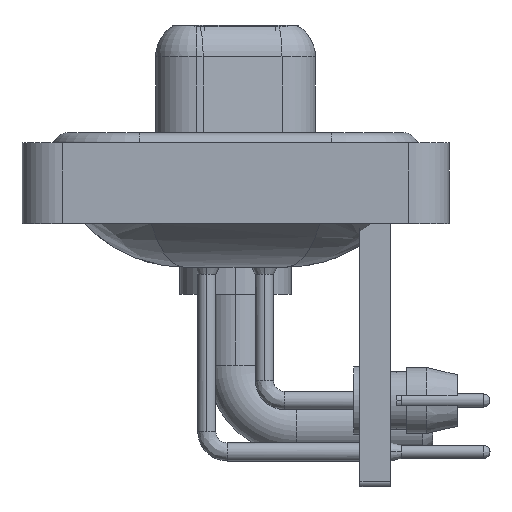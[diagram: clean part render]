
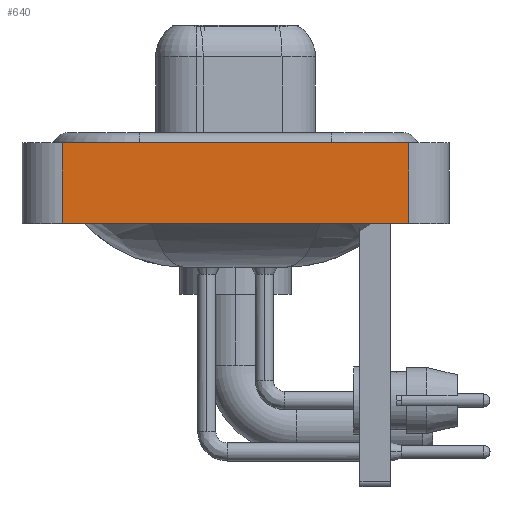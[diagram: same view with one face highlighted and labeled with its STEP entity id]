
A CAD part, left-side view. The second image highlights one B-rep face of the part: STEP entity #640.
In plain terms, the highlighted planar face has unit normal (-1, 0, 0).
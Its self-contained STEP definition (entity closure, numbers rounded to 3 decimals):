
#111 = EDGE_CURVE ( 'NONE', #170, #990, #12064, .T. ) ;
#170 = VERTEX_POINT ( 'NONE', #10015 ) ;
#640 = ADVANCED_FACE ( 'NONE', ( #26534 ), #17726, .T. ) ;
#821 = ORIENTED_EDGE ( 'NONE', *, *, #111, .F. ) ;
#990 = VERTEX_POINT ( 'NONE', #11814 ) ;
#1239 = ORIENTED_EDGE ( 'NONE', *, *, #27075, .T. ) ;
#2678 = VECTOR ( 'NONE', #25420, 1000. ) ;
#3012 = VERTEX_POINT ( 'NONE', #8261 ) ;
#5232 = LINE ( 'NONE', #21174, #9393 ) ;
#5354 = CARTESIAN_POINT ( 'NONE',  ( -7.35, 8.55, -3.6 ) ) ;
#5956 = AXIS2_PLACEMENT_3D ( 'NONE', #17164, #28735, #21721 ) ;
#7904 = VERTEX_POINT ( 'NONE', #26874 ) ;
#8261 = CARTESIAN_POINT ( 'NONE',  ( -7.35, -8.55, -3.6 ) ) ;
#8677 = LINE ( 'NONE', #17750, #10166 ) ;
#8840 = DIRECTION ( 'NONE',  ( 0., -1., 0. ) ) ;
#9393 = VECTOR ( 'NONE', #13995, 1000. ) ;
#10015 = CARTESIAN_POINT ( 'NONE',  ( -7.35, 8.55, -3.6 ) ) ;
#10166 = VECTOR ( 'NONE', #26558, 1000. ) ;
#11035 = LINE ( 'NONE', #19962, #24167 ) ;
#11756 = ORIENTED_EDGE ( 'NONE', *, *, #22994, .F. ) ;
#11814 = CARTESIAN_POINT ( 'NONE',  ( -7.35, 8.55, 0.4 ) ) ;
#12064 = LINE ( 'NONE', #5354, #2678 ) ;
#13995 = DIRECTION ( 'NONE',  ( 0., 0., 1. ) ) ;
#15610 = EDGE_CURVE ( 'NONE', #3012, #7904, #5232, .T. ) ;
#17164 = CARTESIAN_POINT ( 'NONE',  ( -7.35, -8.55, -3.6 ) ) ;
#17726 = PLANE ( 'NONE',  #5956 ) ;
#17750 = CARTESIAN_POINT ( 'NONE',  ( -7.35, -8.55, -3.6 ) ) ;
#19962 = CARTESIAN_POINT ( 'NONE',  ( -7.35, -8.55, 0.4 ) ) ;
#20238 = ORIENTED_EDGE ( 'NONE', *, *, #15610, .T. ) ;
#20846 = EDGE_LOOP ( 'NONE', ( #20238, #11756, #821, #1239 ) ) ;
#21174 = CARTESIAN_POINT ( 'NONE',  ( -7.35, -8.55, -3.6 ) ) ;
#21721 = DIRECTION ( 'NONE',  ( 0., 0., 1. ) ) ;
#22994 = EDGE_CURVE ( 'NONE', #990, #7904, #11035, .T. ) ;
#24167 = VECTOR ( 'NONE', #8840, 1000. ) ;
#25420 = DIRECTION ( 'NONE',  ( 0., 0., 1. ) ) ;
#26534 = FACE_OUTER_BOUND ( 'NONE', #20846, .T. ) ;
#26558 = DIRECTION ( 'NONE',  ( 0., -1., 0. ) ) ;
#26874 = CARTESIAN_POINT ( 'NONE',  ( -7.35, -8.55, 0.4 ) ) ;
#27075 = EDGE_CURVE ( 'NONE', #170, #3012, #8677, .T. ) ;
#28735 = DIRECTION ( 'NONE',  ( -1., 0., 0. ) ) ;
